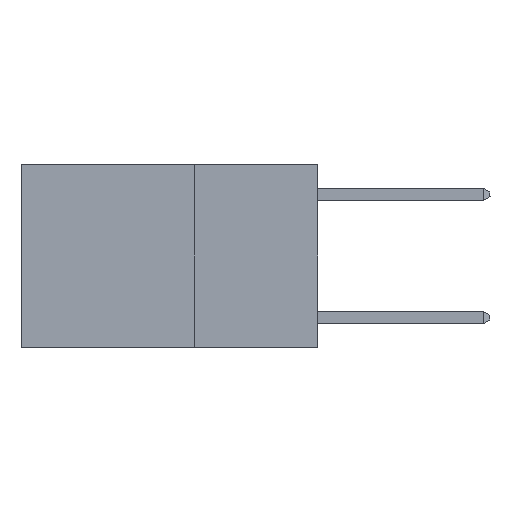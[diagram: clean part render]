
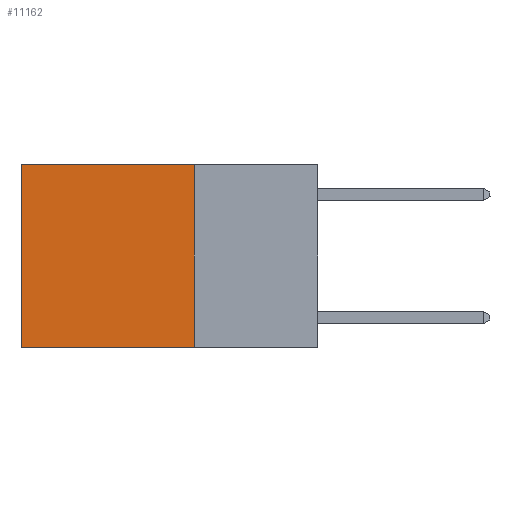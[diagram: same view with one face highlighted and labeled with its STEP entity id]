
A CAD part, left-side view. The second image highlights one B-rep face of the part: STEP entity #11162.
In plain terms, the highlighted planar face has unit normal (-1, 0, 0).
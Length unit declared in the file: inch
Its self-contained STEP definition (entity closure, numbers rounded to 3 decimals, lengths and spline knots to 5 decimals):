
#189 = PLANE ( 'NONE',  #5942 ) ;
#556 = VERTEX_POINT ( 'NONE', #4504 ) ;
#666 = CARTESIAN_POINT ( 'NONE',  ( 0.2625, 0.25, 0. ) ) ;
#811 = EDGE_CURVE ( 'NONE', #556, #7278, #14207, .T. ) ;
#1120 = ORIENTED_EDGE ( 'NONE', *, *, #811, .F. ) ;
#1158 = CARTESIAN_POINT ( 'NONE',  ( 0.2625, 0.6, 0. ) ) ;
#2826 = CARTESIAN_POINT ( 'NONE',  ( 0.2625, 0.25, 0. ) ) ;
#2876 = VECTOR ( 'NONE', #14036, 39.37008 ) ;
#2877 = DIRECTION ( 'NONE',  ( 0., 0., -1. ) ) ;
#2888 = VECTOR ( 'NONE', #2877, 39.37008 ) ;
#4504 = CARTESIAN_POINT ( 'NONE',  ( 0.2625, 0.25, -0.37 ) ) ;
#4851 = CARTESIAN_POINT ( 'NONE',  ( 0.2625, 0.6, 0. ) ) ;
#4949 = CARTESIAN_POINT ( 'NONE',  ( 0.2625, 0.25, 0. ) ) ;
#4951 = ORIENTED_EDGE ( 'NONE', *, *, #10822, .F. ) ;
#5247 = LINE ( 'NONE', #13723, #2888 ) ;
#5583 = ORIENTED_EDGE ( 'NONE', *, *, #14821, .T. ) ;
#5942 = AXIS2_PLACEMENT_3D ( 'NONE', #666, #6333, #11238 ) ;
#6333 = DIRECTION ( 'NONE',  ( 1., 0., 0. ) ) ;
#7278 = VERTEX_POINT ( 'NONE', #12513 ) ;
#7500 = VECTOR ( 'NONE', #11287, 39.37008 ) ;
#8054 = LINE ( 'NONE', #1158, #2876 ) ;
#8221 = CARTESIAN_POINT ( 'NONE',  ( 0.2625, 0.25, -0.37 ) ) ;
#8851 = ORIENTED_EDGE ( 'NONE', *, *, #11873, .T. ) ;
#10822 = EDGE_CURVE ( 'NONE', #14710, #556, #5247, .T. ) ;
#10913 = FACE_OUTER_BOUND ( 'NONE', #13975, .T. ) ;
#11162 = ADVANCED_FACE ( 'NONE', ( #10913 ), #189, .F. ) ;
#11238 = DIRECTION ( 'NONE',  ( 0., 0., -1. ) ) ;
#11287 = DIRECTION ( 'NONE',  ( 0., 1., 0. ) ) ;
#11873 = EDGE_CURVE ( 'NONE', #13710, #7278, #8054, .T. ) ;
#12513 = CARTESIAN_POINT ( 'NONE',  ( 0.2625, 0.6, -0.37 ) ) ;
#12822 = VECTOR ( 'NONE', #12974, 39.37008 ) ;
#12974 = DIRECTION ( 'NONE',  ( 0., 1., 0. ) ) ;
#13527 = LINE ( 'NONE', #2826, #7500 ) ;
#13710 = VERTEX_POINT ( 'NONE', #4851 ) ;
#13723 = CARTESIAN_POINT ( 'NONE',  ( 0.2625, 0.25, 0. ) ) ;
#13975 = EDGE_LOOP ( 'NONE', ( #8851, #1120, #4951, #5583 ) ) ;
#14036 = DIRECTION ( 'NONE',  ( 0., 0., -1. ) ) ;
#14207 = LINE ( 'NONE', #8221, #12822 ) ;
#14710 = VERTEX_POINT ( 'NONE', #4949 ) ;
#14821 = EDGE_CURVE ( 'NONE', #14710, #13710, #13527, .T. ) ;
